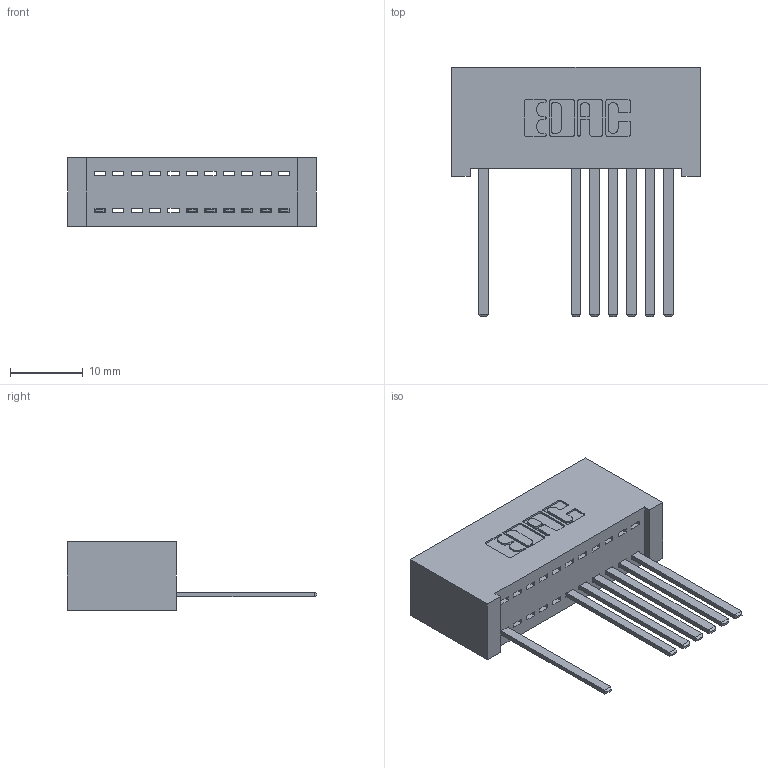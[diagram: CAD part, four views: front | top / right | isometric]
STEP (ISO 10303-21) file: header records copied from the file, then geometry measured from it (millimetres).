
FILE_DESCRIPTION (( 'STEP AP203' ), '1' );
FILE_NAME ('392-011-544-101.STEP', '2018-08-14T21:27:26', ( '' ), ( '' ), 'SwSTEP 2.0', 'SolidWorks 2016', '' );
FILE_SCHEMA (( 'CONFIG_CONTROL_DESIGN' ));
Length unit declared in the file: inch
Products named in the file (3): 392-011-544-101; 342 Part_Lugless; 345-292-001_345-293-144
Assembly tree (8 placements, depth 2):
  392-011-544-101
    342 Part_Lugless
    345-292-001_345-293-144  x7
Bounding box: 34.19 x 34.3 x 9.4 mm (x, y, z)
Volume: 3327.8 mm3; surface area: 4624.8 mm2
Topology: 8 solids, 8 shells, 514 faces, 1549 edges, 1022 vertices
Faces by surface type: plane 376, cylinder 138
Entity records: 10013 total; most frequent: CARTESIAN_POINT 1755, ORIENTED_EDGE 1706, DIRECTION 1527, EDGE_CURVE 853, VECTOR 737, LINE 737, VERTEX_POINT 566, AXIS2_PLACEMENT_3D 395
